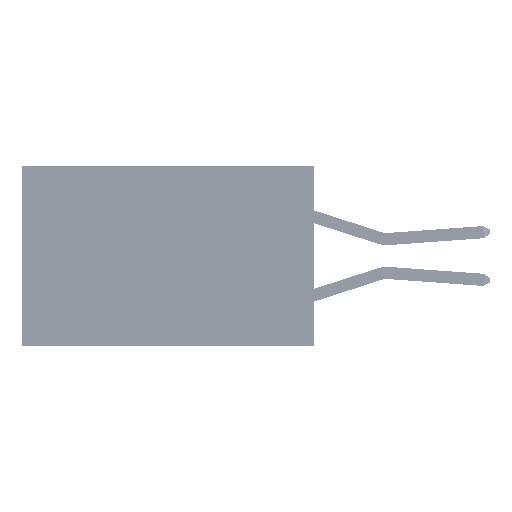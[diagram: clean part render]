
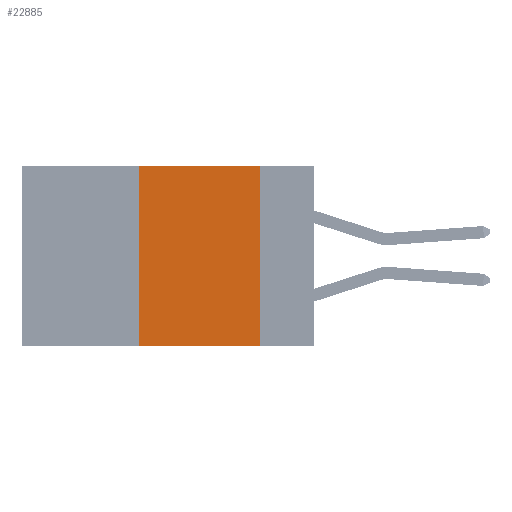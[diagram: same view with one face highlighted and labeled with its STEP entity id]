
A CAD part, left-side view. The second image highlights one B-rep face of the part: STEP entity #22885.
In plain terms, the highlighted planar face has unit normal (-1, 0, 0).
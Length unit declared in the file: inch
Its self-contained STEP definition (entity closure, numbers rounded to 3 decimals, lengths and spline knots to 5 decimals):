
#196 = CARTESIAN_POINT ( 'NONE',  ( 0., 0.11, 0. ) ) ;
#557 = LINE ( 'NONE', #47417, #47721 ) ;
#1093 = DIRECTION ( 'NONE',  ( 0., 0., 1. ) ) ;
#1394 = PLANE ( 'NONE',  #11286 ) ;
#3852 = DIRECTION ( 'NONE',  ( 0., -1., 0. ) ) ;
#6696 = ORIENTED_EDGE ( 'NONE', *, *, #8875, .F. ) ;
#8027 = DIRECTION ( 'NONE',  ( 0., -1., 0. ) ) ;
#8875 = EDGE_CURVE ( 'NONE', #37949, #19482, #49585, .T. ) ;
#10294 = CARTESIAN_POINT ( 'NONE',  ( 0., 0.36, -0.37 ) ) ;
#11286 = AXIS2_PLACEMENT_3D ( 'NONE', #28571, #32144, #32490 ) ;
#13904 = VECTOR ( 'NONE', #8027, 39.37008 ) ;
#18644 = VECTOR ( 'NONE', #3852, 39.37008 ) ;
#19426 = EDGE_CURVE ( 'NONE', #23168, #37949, #557, .T. ) ;
#19482 = VERTEX_POINT ( 'NONE', #20697 ) ;
#19882 = CARTESIAN_POINT ( 'NONE',  ( 0., 0.6, 0. ) ) ;
#20697 = CARTESIAN_POINT ( 'NONE',  ( 0., 0.11, 0. ) ) ;
#20790 = EDGE_LOOP ( 'NONE', ( #38856, #6696, #43751, #48232 ) ) ;
#21176 = FACE_OUTER_BOUND ( 'NONE', #20790, .T. ) ;
#21645 = CARTESIAN_POINT ( 'NONE',  ( 0., 0.36, 0. ) ) ;
#22885 = ADVANCED_FACE ( 'NONE', ( #21176 ), #1394, .F. ) ;
#23168 = VERTEX_POINT ( 'NONE', #10294 ) ;
#25881 = LINE ( 'NONE', #38794, #18644 ) ;
#26114 = CARTESIAN_POINT ( 'NONE',  ( 0., 0.11, -0.37 ) ) ;
#26354 = EDGE_CURVE ( 'NONE', #19482, #38655, #41411, .T. ) ;
#28571 = CARTESIAN_POINT ( 'NONE',  ( 0., 0.6, 0. ) ) ;
#32144 = DIRECTION ( 'NONE',  ( 1., 0., 0. ) ) ;
#32490 = DIRECTION ( 'NONE',  ( 0., 0., -1. ) ) ;
#34533 = DIRECTION ( 'NONE',  ( 0., 0., -1. ) ) ;
#37949 = VERTEX_POINT ( 'NONE', #21645 ) ;
#38655 = VERTEX_POINT ( 'NONE', #26114 ) ;
#38794 = CARTESIAN_POINT ( 'NONE',  ( 0., 0.6, -0.37 ) ) ;
#38856 = ORIENTED_EDGE ( 'NONE', *, *, #26354, .F. ) ;
#41411 = LINE ( 'NONE', #196, #49315 ) ;
#43751 = ORIENTED_EDGE ( 'NONE', *, *, #19426, .F. ) ;
#47417 = CARTESIAN_POINT ( 'NONE',  ( 0., 0.36, 0. ) ) ;
#47721 = VECTOR ( 'NONE', #1093, 39.37008 ) ;
#48232 = ORIENTED_EDGE ( 'NONE', *, *, #49215, .T. ) ;
#49215 = EDGE_CURVE ( 'NONE', #23168, #38655, #25881, .T. ) ;
#49315 = VECTOR ( 'NONE', #34533, 39.37008 ) ;
#49585 = LINE ( 'NONE', #19882, #13904 ) ;
